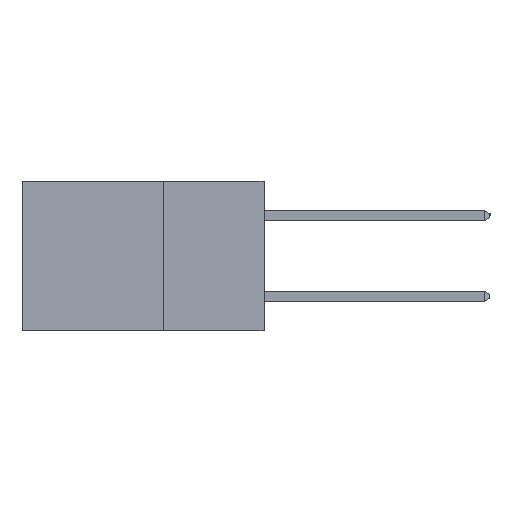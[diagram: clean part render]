
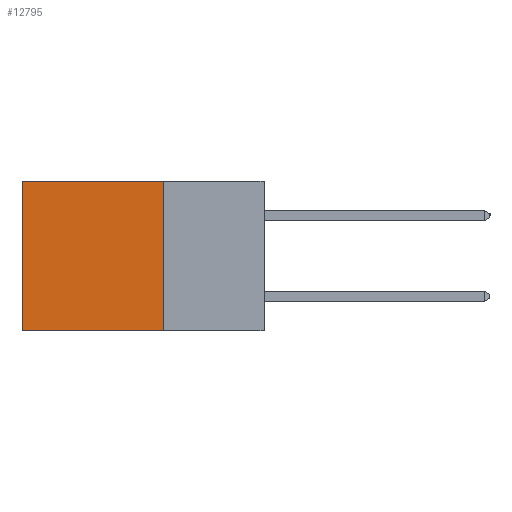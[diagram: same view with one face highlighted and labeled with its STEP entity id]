
A CAD part, left-side view. The second image highlights one B-rep face of the part: STEP entity #12795.
In plain terms, the highlighted planar face has unit normal (-1, 0, 0).
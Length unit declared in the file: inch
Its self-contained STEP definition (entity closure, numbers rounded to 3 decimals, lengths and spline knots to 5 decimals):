
#340 = VECTOR ( 'NONE', #5824, 39.37008 ) ;
#809 = VECTOR ( 'NONE', #829, 39.37008 ) ;
#829 = DIRECTION ( 'NONE',  ( 0., 1., 0. ) ) ;
#1798 = VERTEX_POINT ( 'NONE', #8528 ) ;
#2075 = FACE_OUTER_BOUND ( 'NONE', #10699, .T. ) ;
#2286 = DIRECTION ( 'NONE',  ( 0., 0., -1. ) ) ;
#2584 = VERTEX_POINT ( 'NONE', #9286 ) ;
#2710 = ORIENTED_EDGE ( 'NONE', *, *, #8874, .F. ) ;
#3065 = PLANE ( 'NONE',  #4799 ) ;
#3496 = EDGE_CURVE ( 'NONE', #2584, #5178, #6324, .T. ) ;
#4736 = LINE ( 'NONE', #11078, #809 ) ;
#4799 = AXIS2_PLACEMENT_3D ( 'NONE', #12473, #5172, #9253 ) ;
#4876 = ORIENTED_EDGE ( 'NONE', *, *, #7343, .F. ) ;
#5172 = DIRECTION ( 'NONE',  ( 1., 0., 0. ) ) ;
#5178 = VERTEX_POINT ( 'NONE', #11934 ) ;
#5539 = VECTOR ( 'NONE', #11405, 39.37008 ) ;
#5824 = DIRECTION ( 'NONE',  ( 0., 0., -1. ) ) ;
#6063 = CARTESIAN_POINT ( 'NONE',  ( 0.2615, 0.25, 0. ) ) ;
#6324 = LINE ( 'NONE', #6063, #5539 ) ;
#6341 = CARTESIAN_POINT ( 'NONE',  ( 0.2615, 0.25, -0.37 ) ) ;
#6689 = VECTOR ( 'NONE', #2286, 39.37008 ) ;
#7343 = EDGE_CURVE ( 'NONE', #2584, #10513, #11425, .T. ) ;
#7960 = LINE ( 'NONE', #13128, #340 ) ;
#8091 = CARTESIAN_POINT ( 'NONE',  ( 0.2615, 0.25, -0.37 ) ) ;
#8528 = CARTESIAN_POINT ( 'NONE',  ( 0.2615, 0.6, -0.37 ) ) ;
#8874 = EDGE_CURVE ( 'NONE', #10513, #1798, #4736, .T. ) ;
#9087 = ORIENTED_EDGE ( 'NONE', *, *, #9820, .T. ) ;
#9253 = DIRECTION ( 'NONE',  ( 0., 0., -1. ) ) ;
#9286 = CARTESIAN_POINT ( 'NONE',  ( 0.2615, 0.25, 0. ) ) ;
#9820 = EDGE_CURVE ( 'NONE', #5178, #1798, #7960, .T. ) ;
#10513 = VERTEX_POINT ( 'NONE', #8091 ) ;
#10529 = ORIENTED_EDGE ( 'NONE', *, *, #3496, .T. ) ;
#10699 = EDGE_LOOP ( 'NONE', ( #9087, #2710, #4876, #10529 ) ) ;
#11078 = CARTESIAN_POINT ( 'NONE',  ( 0.2615, 0.25, -0.37 ) ) ;
#11405 = DIRECTION ( 'NONE',  ( 0., 1., 0. ) ) ;
#11425 = LINE ( 'NONE', #6341, #6689 ) ;
#11934 = CARTESIAN_POINT ( 'NONE',  ( 0.2615, 0.6, 0. ) ) ;
#12473 = CARTESIAN_POINT ( 'NONE',  ( 0.2615, 0.25, -0.37 ) ) ;
#12795 = ADVANCED_FACE ( 'NONE', ( #2075 ), #3065, .F. ) ;
#13128 = CARTESIAN_POINT ( 'NONE',  ( 0.2615, 0.6, -0.37 ) ) ;
